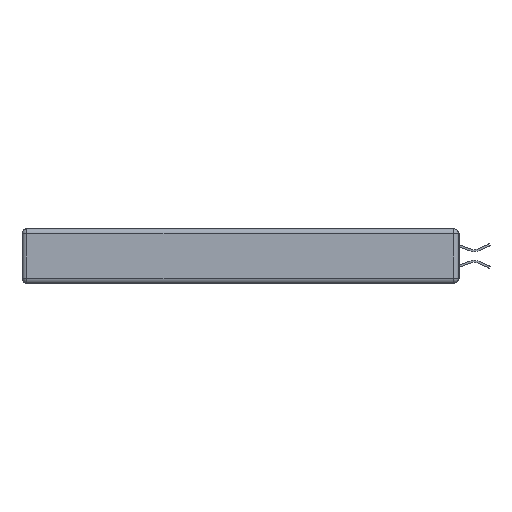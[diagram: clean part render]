
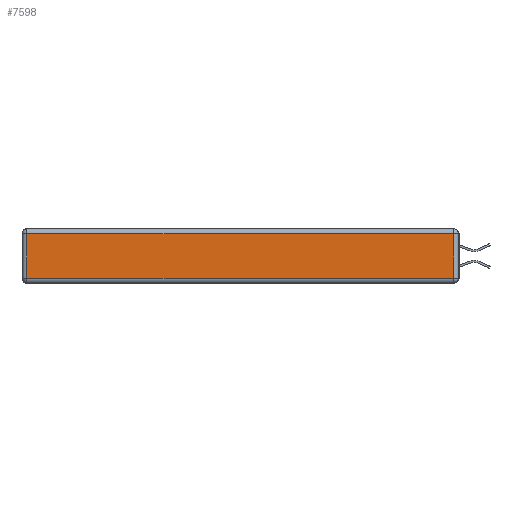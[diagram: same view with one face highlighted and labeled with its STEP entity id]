
A CAD part, left-side view. The second image highlights one B-rep face of the part: STEP entity #7598.
In plain terms, the highlighted planar face has unit normal (-1, 0, 0).
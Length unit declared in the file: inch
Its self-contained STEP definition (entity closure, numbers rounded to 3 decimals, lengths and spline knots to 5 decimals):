
#1243 = CARTESIAN_POINT ( 'NONE',  ( 0., 0., -0.313 ) ) ;
#1411 = DIRECTION ( 'NONE',  ( 0., 0., 1. ) ) ;
#1656 = LINE ( 'NONE', #15631, #26361 ) ;
#1898 = EDGE_CURVE ( 'NONE', #19306, #25192, #1656, .T. ) ;
#3018 = CARTESIAN_POINT ( 'NONE',  ( 0., 0.03, -0.03 ) ) ;
#3297 = CARTESIAN_POINT ( 'NONE',  ( 0., 2.72, -0.03 ) ) ;
#3469 = EDGE_CURVE ( 'NONE', #27817, #17602, #9601, .T. ) ;
#4442 = EDGE_LOOP ( 'NONE', ( #9214, #6242, #7786, #5023 ) ) ;
#4715 = VECTOR ( 'NONE', #1411, 39.37008 ) ;
#5023 = ORIENTED_EDGE ( 'NONE', *, *, #22636, .T. ) ;
#6242 = ORIENTED_EDGE ( 'NONE', *, *, #18453, .T. ) ;
#7598 = ADVANCED_FACE ( 'NONE', ( #8852 ), #21593, .T. ) ;
#7786 = ORIENTED_EDGE ( 'NONE', *, *, #1898, .T. ) ;
#8125 = DIRECTION ( 'NONE',  ( 0., 0., 1. ) ) ;
#8469 = DIRECTION ( 'NONE',  ( 0., 1., 0. ) ) ;
#8852 = FACE_OUTER_BOUND ( 'NONE', #4442, .T. ) ;
#9214 = ORIENTED_EDGE ( 'NONE', *, *, #3469, .T. ) ;
#9601 = LINE ( 'NONE', #1243, #15316 ) ;
#9876 = DIRECTION ( 'NONE',  ( 0., -1., 0. ) ) ;
#10065 = LINE ( 'NONE', #22873, #19696 ) ;
#10277 = DIRECTION ( 'NONE',  ( -1., 0., 0. ) ) ;
#15316 = VECTOR ( 'NONE', #9876, 39.37008 ) ;
#15631 = CARTESIAN_POINT ( 'NONE',  ( 0., 2.75, -0.03 ) ) ;
#16725 = LINE ( 'NONE', #17278, #4715 ) ;
#17278 = CARTESIAN_POINT ( 'NONE',  ( 0., 0.03, -0.343 ) ) ;
#17602 = VERTEX_POINT ( 'NONE', #25960 ) ;
#18453 = EDGE_CURVE ( 'NONE', #17602, #19306, #16725, .T. ) ;
#19306 = VERTEX_POINT ( 'NONE', #3018 ) ;
#19696 = VECTOR ( 'NONE', #22689, 39.37008 ) ;
#21593 = PLANE ( 'NONE',  #22474 ) ;
#22474 = AXIS2_PLACEMENT_3D ( 'NONE', #26221, #10277, #8125 ) ;
#22636 = EDGE_CURVE ( 'NONE', #25192, #27817, #10065, .T. ) ;
#22689 = DIRECTION ( 'NONE',  ( 0., 0., -1. ) ) ;
#22873 = CARTESIAN_POINT ( 'NONE',  ( 0., 2.72, -0.343 ) ) ;
#25192 = VERTEX_POINT ( 'NONE', #3297 ) ;
#25752 = CARTESIAN_POINT ( 'NONE',  ( 0., 2.72, -0.313 ) ) ;
#25960 = CARTESIAN_POINT ( 'NONE',  ( 0., 0.03, -0.313 ) ) ;
#26221 = CARTESIAN_POINT ( 'NONE',  ( 0., 0., -0.343 ) ) ;
#26361 = VECTOR ( 'NONE', #8469, 39.37008 ) ;
#27817 = VERTEX_POINT ( 'NONE', #25752 ) ;
